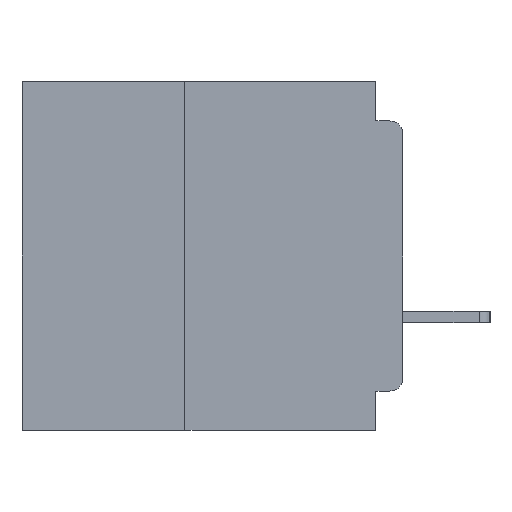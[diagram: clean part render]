
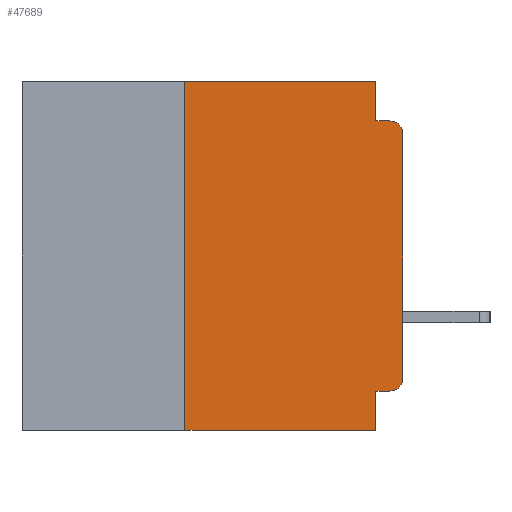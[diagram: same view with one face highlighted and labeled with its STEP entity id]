
A CAD part, left-side view. The second image highlights one B-rep face of the part: STEP entity #47689.
In plain terms, the highlighted planar face has unit normal (-1, 0, 0).
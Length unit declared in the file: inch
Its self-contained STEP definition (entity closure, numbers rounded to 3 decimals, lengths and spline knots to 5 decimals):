
#20 = ORIENTED_EDGE ( 'NONE', *, *, #25157, .F. ) ;
#686 = CARTESIAN_POINT ( 'NONE',  ( 0., 0.015, -0.355 ) ) ;
#940 = ORIENTED_EDGE ( 'NONE', *, *, #5468, .F. ) ;
#950 = VECTOR ( 'NONE', #21263, 39.37008 ) ;
#1864 = CARTESIAN_POINT ( 'NONE',  ( 0., 0.015, -0.06 ) ) ;
#2964 = DIRECTION ( 'NONE',  ( 0., -1., 0. ) ) ;
#4048 = CARTESIAN_POINT ( 'NONE',  ( 0., 0., -0.06 ) ) ;
#4978 = VECTOR ( 'NONE', #2964, 39.37008 ) ;
#5468 = EDGE_CURVE ( 'NONE', #42814, #7904, #25879, .T. ) ;
#6279 = DIRECTION ( 'NONE',  ( 0., 0., -1. ) ) ;
#6657 = EDGE_CURVE ( 'NONE', #28772, #49366, #44298, .T. ) ;
#6940 = VERTEX_POINT ( 'NONE', #4048 ) ;
#7904 = VERTEX_POINT ( 'NONE', #44928 ) ;
#8282 = FACE_OUTER_BOUND ( 'NONE', #16887, .T. ) ;
#8403 = DIRECTION ( 'NONE',  ( -1., 0., 0. ) ) ;
#8405 = DIRECTION ( 'NONE',  ( 0., 1., 0. ) ) ;
#9104 = DIRECTION ( 'NONE',  ( 0., 0., 1. ) ) ;
#10445 = CARTESIAN_POINT ( 'NONE',  ( 0., 0.031, -0.045 ) ) ;
#11377 = DIRECTION ( 'NONE',  ( 0., -1., 0. ) ) ;
#12095 = AXIS2_PLACEMENT_3D ( 'NONE', #34821, #8403, #39253 ) ;
#13522 = VECTOR ( 'NONE', #9104, 39.37008 ) ;
#13750 = CARTESIAN_POINT ( 'NONE',  ( 0., 0.25, -0.4 ) ) ;
#14174 = VECTOR ( 'NONE', #11377, 39.37008 ) ;
#14343 = LINE ( 'NONE', #17260, #24671 ) ;
#14564 = ORIENTED_EDGE ( 'NONE', *, *, #18048, .T. ) ;
#14662 = VERTEX_POINT ( 'NONE', #22216 ) ;
#15780 = CARTESIAN_POINT ( 'NONE',  ( 0., 0., -0.045 ) ) ;
#16887 = EDGE_LOOP ( 'NONE', ( #51224, #41864, #940, #20, #50225, #31023, #14564, #23951, #19386, #47498 ) ) ;
#17260 = CARTESIAN_POINT ( 'NONE',  ( 0., 0., -0.355 ) ) ;
#17823 = CARTESIAN_POINT ( 'NONE',  ( 0., 0.031, 0. ) ) ;
#18048 = EDGE_CURVE ( 'NONE', #41535, #51096, #40183, .T. ) ;
#19386 = ORIENTED_EDGE ( 'NONE', *, *, #35567, .F. ) ;
#20553 = CARTESIAN_POINT ( 'NONE',  ( 0., 0.25, -0.4 ) ) ;
#21263 = DIRECTION ( 'NONE',  ( 0., 0., -1. ) ) ;
#21645 = VERTEX_POINT ( 'NONE', #48447 ) ;
#22216 = CARTESIAN_POINT ( 'NONE',  ( 0., 0.031, -0.355 ) ) ;
#22257 = DIRECTION ( 'NONE',  ( 0., 0., -1. ) ) ;
#23951 = ORIENTED_EDGE ( 'NONE', *, *, #32992, .F. ) ;
#24292 = DIRECTION ( 'NONE',  ( 1., 0., 0. ) ) ;
#24671 = VECTOR ( 'NONE', #8405, 39.37008 ) ;
#24928 = CARTESIAN_POINT ( 'NONE',  ( 0., 0.437, -0.4 ) ) ;
#25157 = EDGE_CURVE ( 'NONE', #49366, #42814, #30161, .T. ) ;
#25224 = LINE ( 'NONE', #35523, #13522 ) ;
#25879 = LINE ( 'NONE', #15780, #14174 ) ;
#26763 = AXIS2_PLACEMENT_3D ( 'NONE', #1864, #32696, #6279 ) ;
#27247 = CARTESIAN_POINT ( 'NONE',  ( 0., 0.25, 0. ) ) ;
#28542 = CARTESIAN_POINT ( 'NONE',  ( 0., 0.437, 0. ) ) ;
#28772 = VERTEX_POINT ( 'NONE', #27247 ) ;
#29945 = VERTEX_POINT ( 'NONE', #686 ) ;
#30161 = LINE ( 'NONE', #17823, #39145 ) ;
#30469 = EDGE_CURVE ( 'NONE', #41535, #28772, #31017, .T. ) ;
#31017 = LINE ( 'NONE', #20553, #52910 ) ;
#31023 = ORIENTED_EDGE ( 'NONE', *, *, #30469, .F. ) ;
#31249 = VECTOR ( 'NONE', #32977, 39.37008 ) ;
#32696 = DIRECTION ( 'NONE',  ( -1., 0., 0. ) ) ;
#32977 = DIRECTION ( 'NONE',  ( 0., -1., 0. ) ) ;
#32992 = EDGE_CURVE ( 'NONE', #14662, #51096, #47735, .T. ) ;
#34397 = CARTESIAN_POINT ( 'NONE',  ( 0., 0.031, -0.4 ) ) ;
#34821 = CARTESIAN_POINT ( 'NONE',  ( 0., 0.015, -0.34 ) ) ;
#35523 = CARTESIAN_POINT ( 'NONE',  ( 0., 0., 0. ) ) ;
#35567 = EDGE_CURVE ( 'NONE', #29945, #14662, #14343, .T. ) ;
#39145 = VECTOR ( 'NONE', #22257, 39.37008 ) ;
#39253 = DIRECTION ( 'NONE',  ( 0., 0., -1. ) ) ;
#40183 = LINE ( 'NONE', #24928, #4978 ) ;
#40775 = EDGE_CURVE ( 'NONE', #29945, #21645, #54064, .T. ) ;
#41535 = VERTEX_POINT ( 'NONE', #13750 ) ;
#41864 = ORIENTED_EDGE ( 'NONE', *, *, #48251, .T. ) ;
#42301 = CARTESIAN_POINT ( 'NONE',  ( 0., 0.031, -0.4 ) ) ;
#42814 = VERTEX_POINT ( 'NONE', #10445 ) ;
#43667 = AXIS2_PLACEMENT_3D ( 'NONE', #28542, #24292, #54937 ) ;
#44298 = LINE ( 'NONE', #50390, #31249 ) ;
#44928 = CARTESIAN_POINT ( 'NONE',  ( 0., 0.015, -0.045 ) ) ;
#45616 = CARTESIAN_POINT ( 'NONE',  ( 0., 0.031, 0. ) ) ;
#46878 = DIRECTION ( 'NONE',  ( 0., 0., 1. ) ) ;
#47498 = ORIENTED_EDGE ( 'NONE', *, *, #40775, .T. ) ;
#47689 = ADVANCED_FACE ( 'NONE', ( #8282 ), #50537, .F. ) ;
#47735 = LINE ( 'NONE', #34397, #950 ) ;
#48103 = CIRCLE ( 'NONE', #26763, 0.015 ) ;
#48251 = EDGE_CURVE ( 'NONE', #6940, #7904, #48103, .T. ) ;
#48447 = CARTESIAN_POINT ( 'NONE',  ( 0., 0., -0.34 ) ) ;
#49366 = VERTEX_POINT ( 'NONE', #45616 ) ;
#50168 = EDGE_CURVE ( 'NONE', #21645, #6940, #25224, .T. ) ;
#50225 = ORIENTED_EDGE ( 'NONE', *, *, #6657, .F. ) ;
#50390 = CARTESIAN_POINT ( 'NONE',  ( 0., 0.437, 0. ) ) ;
#50537 = PLANE ( 'NONE',  #43667 ) ;
#51096 = VERTEX_POINT ( 'NONE', #42301 ) ;
#51224 = ORIENTED_EDGE ( 'NONE', *, *, #50168, .T. ) ;
#52910 = VECTOR ( 'NONE', #46878, 39.37008 ) ;
#54064 = CIRCLE ( 'NONE', #12095, 0.015 ) ;
#54937 = DIRECTION ( 'NONE',  ( 0., 0., -1. ) ) ;
